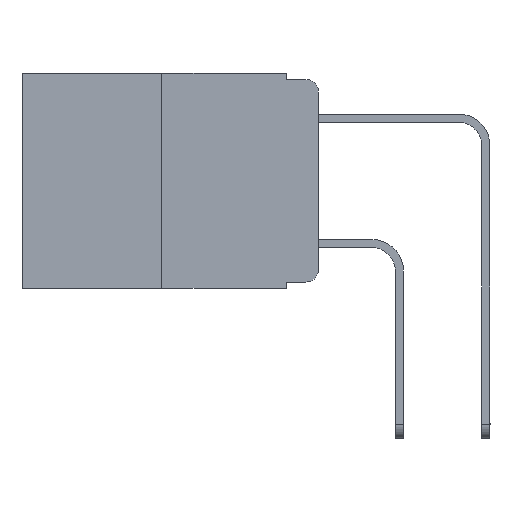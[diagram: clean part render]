
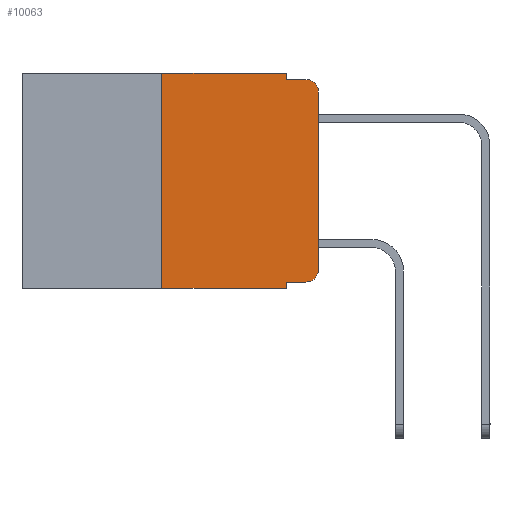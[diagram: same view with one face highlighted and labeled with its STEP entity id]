
A CAD part, left-side view. The second image highlights one B-rep face of the part: STEP entity #10063.
In plain terms, the highlighted planar face has unit normal (-1, 0, 0).
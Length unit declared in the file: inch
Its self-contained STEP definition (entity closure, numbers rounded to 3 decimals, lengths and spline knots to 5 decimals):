
#150 = DIRECTION ( 'NONE',  ( 0., 0., 1. ) ) ;
#227 = EDGE_CURVE ( 'NONE', #10150, #7231, #3157, .T. ) ;
#542 = DIRECTION ( 'NONE',  ( 0., -1., 0. ) ) ;
#637 = VERTEX_POINT ( 'NONE', #11436 ) ;
#1553 = DIRECTION ( 'NONE',  ( 0., 0., -1. ) ) ;
#1635 = CARTESIAN_POINT ( 'NONE',  ( 0., 0.051, -0.333 ) ) ;
#1727 = EDGE_CURVE ( 'NONE', #637, #11603, #2995, .T. ) ;
#1952 = VECTOR ( 'NONE', #542, 39.37008 ) ;
#2097 = VECTOR ( 'NONE', #7381, 39.37008 ) ;
#2591 = AXIS2_PLACEMENT_3D ( 'NONE', #2655, #4825, #1553 ) ;
#2655 = CARTESIAN_POINT ( 'NONE',  ( 0., 0.473, 0. ) ) ;
#2681 = LINE ( 'NONE', #6199, #2097 ) ;
#2723 = DIRECTION ( 'NONE',  ( -1., 0., 0. ) ) ;
#2729 = CARTESIAN_POINT ( 'NONE',  ( 0., 0., 0. ) ) ;
#2731 = DIRECTION ( 'NONE',  ( 0., 0., -1. ) ) ;
#2925 = ORIENTED_EDGE ( 'NONE', *, *, #11327, .T. ) ;
#2962 = DIRECTION ( 'NONE',  ( 0., 0., -1. ) ) ;
#2994 = VECTOR ( 'NONE', #9964, 39.37008 ) ;
#2995 = LINE ( 'NONE', #11367, #3938 ) ;
#3157 = LINE ( 'NONE', #15299, #12378 ) ;
#3189 = CARTESIAN_POINT ( 'NONE',  ( 0., 0.051, -0.01 ) ) ;
#3284 = VERTEX_POINT ( 'NONE', #10483 ) ;
#3593 = CIRCLE ( 'NONE', #4824, 0.02 ) ;
#3907 = ORIENTED_EDGE ( 'NONE', *, *, #10060, .T. ) ;
#3925 = DIRECTION ( 'NONE',  ( 0., 0., -1. ) ) ;
#3938 = VECTOR ( 'NONE', #3925, 39.37008 ) ;
#3958 = ORIENTED_EDGE ( 'NONE', *, *, #10283, .F. ) ;
#3975 = EDGE_LOOP ( 'NONE', ( #3907, #2925, #9340, #10241, #3958, #12273, #13786, #12576, #12525, #4520 ) ) ;
#4113 = VERTEX_POINT ( 'NONE', #8654 ) ;
#4520 = ORIENTED_EDGE ( 'NONE', *, *, #14654, .T. ) ;
#4646 = CARTESIAN_POINT ( 'NONE',  ( 0., 0.473, -0.343 ) ) ;
#4824 = AXIS2_PLACEMENT_3D ( 'NONE', #10883, #12060, #2731 ) ;
#4825 = DIRECTION ( 'NONE',  ( 1., 0., 0. ) ) ;
#5187 = CARTESIAN_POINT ( 'NONE',  ( 0., 0.051, -0.01 ) ) ;
#5205 = VECTOR ( 'NONE', #6222, 39.37008 ) ;
#5297 = CARTESIAN_POINT ( 'NONE',  ( 0., 0.051, -0.333 ) ) ;
#5416 = DIRECTION ( 'NONE',  ( 0., 0., -1. ) ) ;
#5971 = CARTESIAN_POINT ( 'NONE',  ( 0., 0.473, 0. ) ) ;
#6140 = EDGE_CURVE ( 'NONE', #11603, #3284, #6749, .T. ) ;
#6199 = CARTESIAN_POINT ( 'NONE',  ( 0., 0.25, 0. ) ) ;
#6222 = DIRECTION ( 'NONE',  ( 0., -1., 0. ) ) ;
#6321 = PLANE ( 'NONE',  #2591 ) ;
#6604 = AXIS2_PLACEMENT_3D ( 'NONE', #12434, #2723, #2962 ) ;
#6749 = LINE ( 'NONE', #5187, #2994 ) ;
#7231 = VERTEX_POINT ( 'NONE', #7397 ) ;
#7381 = DIRECTION ( 'NONE',  ( 0., 0., 1. ) ) ;
#7397 = CARTESIAN_POINT ( 'NONE',  ( 0., 0.051, -0.343 ) ) ;
#8312 = EDGE_CURVE ( 'NONE', #10150, #9287, #12432, .T. ) ;
#8446 = FACE_OUTER_BOUND ( 'NONE', #3975, .T. ) ;
#8590 = VERTEX_POINT ( 'NONE', #14459 ) ;
#8644 = EDGE_CURVE ( 'NONE', #14691, #7231, #15407, .T. ) ;
#8654 = CARTESIAN_POINT ( 'NONE',  ( 0., 0., -0.03 ) ) ;
#9287 = VERTEX_POINT ( 'NONE', #15062 ) ;
#9340 = ORIENTED_EDGE ( 'NONE', *, *, #6140, .F. ) ;
#9497 = LINE ( 'NONE', #5971, #10089 ) ;
#9929 = CARTESIAN_POINT ( 'NONE',  ( 0., 0.25, 0. ) ) ;
#9964 = DIRECTION ( 'NONE',  ( 0., -1., 0. ) ) ;
#10060 = EDGE_CURVE ( 'NONE', #8590, #4113, #13385, .T. ) ;
#10063 = ADVANCED_FACE ( 'NONE', ( #8446 ), #6321, .F. ) ;
#10089 = VECTOR ( 'NONE', #15394, 39.37008 ) ;
#10150 = VERTEX_POINT ( 'NONE', #1635 ) ;
#10241 = ORIENTED_EDGE ( 'NONE', *, *, #1727, .F. ) ;
#10283 = EDGE_CURVE ( 'NONE', #14306, #637, #9497, .T. ) ;
#10483 = CARTESIAN_POINT ( 'NONE',  ( 0., 0.02, -0.01 ) ) ;
#10883 = CARTESIAN_POINT ( 'NONE',  ( 0., 0.02, -0.03 ) ) ;
#11176 = CARTESIAN_POINT ( 'NONE',  ( 0., 0.25, -0.343 ) ) ;
#11327 = EDGE_CURVE ( 'NONE', #4113, #3284, #3593, .T. ) ;
#11367 = CARTESIAN_POINT ( 'NONE',  ( 0., 0.051, 0. ) ) ;
#11436 = CARTESIAN_POINT ( 'NONE',  ( 0., 0.051, 0. ) ) ;
#11603 = VERTEX_POINT ( 'NONE', #3189 ) ;
#12060 = DIRECTION ( 'NONE',  ( -1., 0., 0. ) ) ;
#12269 = EDGE_CURVE ( 'NONE', #14691, #14306, #2681, .T. ) ;
#12273 = ORIENTED_EDGE ( 'NONE', *, *, #12269, .F. ) ;
#12378 = VECTOR ( 'NONE', #5416, 39.37008 ) ;
#12432 = LINE ( 'NONE', #5297, #1952 ) ;
#12434 = CARTESIAN_POINT ( 'NONE',  ( 0., 0.02, -0.313 ) ) ;
#12525 = ORIENTED_EDGE ( 'NONE', *, *, #8312, .T. ) ;
#12576 = ORIENTED_EDGE ( 'NONE', *, *, #227, .F. ) ;
#13371 = CIRCLE ( 'NONE', #6604, 0.02 ) ;
#13385 = LINE ( 'NONE', #2729, #13848 ) ;
#13786 = ORIENTED_EDGE ( 'NONE', *, *, #8644, .T. ) ;
#13848 = VECTOR ( 'NONE', #150, 39.37008 ) ;
#14306 = VERTEX_POINT ( 'NONE', #9929 ) ;
#14459 = CARTESIAN_POINT ( 'NONE',  ( 0., 0., -0.313 ) ) ;
#14654 = EDGE_CURVE ( 'NONE', #9287, #8590, #13371, .T. ) ;
#14691 = VERTEX_POINT ( 'NONE', #11176 ) ;
#15062 = CARTESIAN_POINT ( 'NONE',  ( 0., 0.02, -0.333 ) ) ;
#15299 = CARTESIAN_POINT ( 'NONE',  ( 0., 0.051, 0. ) ) ;
#15394 = DIRECTION ( 'NONE',  ( 0., -1., 0. ) ) ;
#15407 = LINE ( 'NONE', #4646, #5205 ) ;
